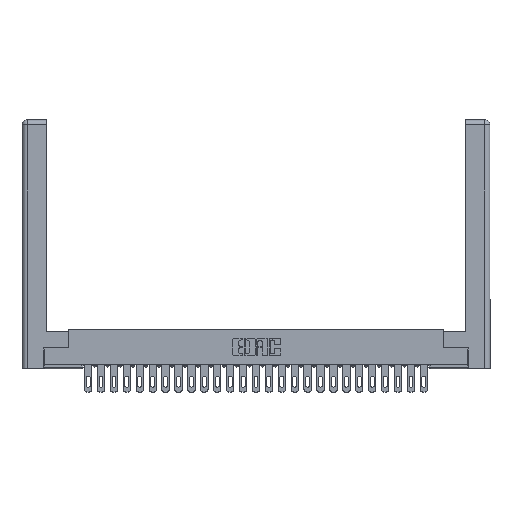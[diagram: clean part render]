
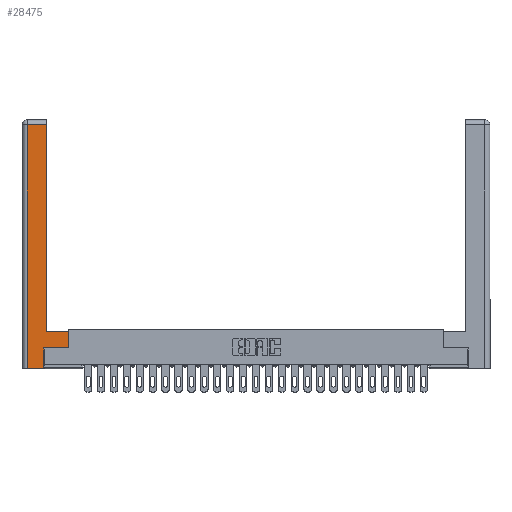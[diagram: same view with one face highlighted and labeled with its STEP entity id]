
A CAD part, top view. The second image highlights one B-rep face of the part: STEP entity #28475.
In plain terms, the highlighted planar face has unit normal (0, 0, 1).
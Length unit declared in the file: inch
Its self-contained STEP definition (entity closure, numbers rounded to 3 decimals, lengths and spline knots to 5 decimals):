
#11 = DIRECTION ( 'NONE',  ( 0., 1., 0. ) ) ;
#244 = CARTESIAN_POINT ( 'NONE',  ( 0.565, 0.245, 0. ) ) ;
#382 = ORIENTED_EDGE ( 'NONE', *, *, #28172, .T. ) ;
#699 = EDGE_CURVE ( 'NONE', #25118, #24480, #10705, .T. ) ;
#803 = CARTESIAN_POINT ( 'NONE',  ( 0.265, 0., 0. ) ) ;
#1502 = LINE ( 'NONE', #10168, #19481 ) ;
#2156 = VERTEX_POINT ( 'NONE', #7500 ) ;
#2638 = DIRECTION ( 'NONE',  ( 0., 0., -1. ) ) ;
#2921 = DIRECTION ( 'NONE',  ( -1., 0., 0. ) ) ;
#2941 = VECTOR ( 'NONE', #20913, 39.37008 ) ;
#3343 = VECTOR ( 'NONE', #12584, 39.37008 ) ;
#3544 = VECTOR ( 'NONE', #11, 39.37008 ) ;
#4178 = VECTOR ( 'NONE', #9614, 39.37008 ) ;
#4421 = LINE ( 'NONE', #15531, #13533 ) ;
#4644 = ORIENTED_EDGE ( 'NONE', *, *, #18650, .T. ) ;
#5301 = EDGE_CURVE ( 'NONE', #11600, #13776, #1502, .T. ) ;
#6294 = CARTESIAN_POINT ( 'NONE',  ( 0.565, 0.45, 0. ) ) ;
#6384 = CARTESIAN_POINT ( 'NONE',  ( 0.565, 0.45, 0. ) ) ;
#7223 = CARTESIAN_POINT ( 'NONE',  ( 0.295, 2.94, 0. ) ) ;
#7500 = CARTESIAN_POINT ( 'NONE',  ( 0.295, 0.45, 0. ) ) ;
#7998 = EDGE_CURVE ( 'NONE', #13469, #25118, #9651, .T. ) ;
#9614 = DIRECTION ( 'NONE',  ( 1., 0., 0. ) ) ;
#9651 = LINE ( 'NONE', #14152, #2941 ) ;
#10168 = CARTESIAN_POINT ( 'NONE',  ( 0.0615, 0., 0. ) ) ;
#10188 = AXIS2_PLACEMENT_3D ( 'NONE', #18360, #2638, #2921 ) ;
#10304 = CARTESIAN_POINT ( 'NONE',  ( 0.0615, 2.94, 0. ) ) ;
#10531 = VERTEX_POINT ( 'NONE', #7223 ) ;
#10705 = LINE ( 'NONE', #15296, #27817 ) ;
#11600 = VERTEX_POINT ( 'NONE', #10304 ) ;
#11806 = LINE ( 'NONE', #803, #4178 ) ;
#11919 = EDGE_CURVE ( 'NONE', #2156, #10531, #16897, .T. ) ;
#12286 = ORIENTED_EDGE ( 'NONE', *, *, #5301, .T. ) ;
#12584 = DIRECTION ( 'NONE',  ( 0., 1., 0. ) ) ;
#13469 = VERTEX_POINT ( 'NONE', #24839 ) ;
#13533 = VECTOR ( 'NONE', #19833, 39.37008 ) ;
#13776 = VERTEX_POINT ( 'NONE', #27354 ) ;
#14061 = VERTEX_POINT ( 'NONE', #6294 ) ;
#14091 = EDGE_CURVE ( 'NONE', #10531, #11600, #4421, .T. ) ;
#14152 = CARTESIAN_POINT ( 'NONE',  ( 0.265, 0.245, 0. ) ) ;
#14636 = ORIENTED_EDGE ( 'NONE', *, *, #14091, .T. ) ;
#14652 = DIRECTION ( 'NONE',  ( 0., -1., 0. ) ) ;
#15237 = EDGE_LOOP ( 'NONE', ( #25276, #14636, #12286, #382, #27289, #16051, #26134, #4644 ) ) ;
#15296 = CARTESIAN_POINT ( 'NONE',  ( 0.565, 0.245, 0. ) ) ;
#15531 = CARTESIAN_POINT ( 'NONE',  ( 0.0615, 2.94, 0. ) ) ;
#16051 = ORIENTED_EDGE ( 'NONE', *, *, #699, .T. ) ;
#16897 = LINE ( 'NONE', #25797, #3343 ) ;
#18360 = CARTESIAN_POINT ( 'NONE',  ( 0., 0., 0. ) ) ;
#18499 = PLANE ( 'NONE',  #10188 ) ;
#18650 = EDGE_CURVE ( 'NONE', #14061, #2156, #25901, .T. ) ;
#19476 = DIRECTION ( 'NONE',  ( 1., 0., 0. ) ) ;
#19481 = VECTOR ( 'NONE', #14652, 39.37008 ) ;
#19833 = DIRECTION ( 'NONE',  ( -1., 0., 0. ) ) ;
#20109 = FACE_OUTER_BOUND ( 'NONE', #15237, .T. ) ;
#20913 = DIRECTION ( 'NONE',  ( 0., 1., 0. ) ) ;
#21135 = CARTESIAN_POINT ( 'NONE',  ( 0.265, 0.245, 0. ) ) ;
#21331 = DIRECTION ( 'NONE',  ( -1., 0., 0. ) ) ;
#23773 = CARTESIAN_POINT ( 'NONE',  ( 0.295, 0.45, 0. ) ) ;
#24404 = LINE ( 'NONE', #6384, #3544 ) ;
#24480 = VERTEX_POINT ( 'NONE', #244 ) ;
#24839 = CARTESIAN_POINT ( 'NONE',  ( 0.265, 0., 0. ) ) ;
#25118 = VERTEX_POINT ( 'NONE', #21135 ) ;
#25229 = EDGE_CURVE ( 'NONE', #24480, #14061, #24404, .T. ) ;
#25276 = ORIENTED_EDGE ( 'NONE', *, *, #11919, .T. ) ;
#25570 = VECTOR ( 'NONE', #21331, 39.37008 ) ;
#25797 = CARTESIAN_POINT ( 'NONE',  ( 0.295, 3., 0. ) ) ;
#25901 = LINE ( 'NONE', #23773, #25570 ) ;
#26134 = ORIENTED_EDGE ( 'NONE', *, *, #25229, .T. ) ;
#27289 = ORIENTED_EDGE ( 'NONE', *, *, #7998, .T. ) ;
#27354 = CARTESIAN_POINT ( 'NONE',  ( 0.0615, 0., 0. ) ) ;
#27817 = VECTOR ( 'NONE', #19476, 39.37008 ) ;
#28172 = EDGE_CURVE ( 'NONE', #13776, #13469, #11806, .T. ) ;
#28475 = ADVANCED_FACE ( 'NONE', ( #20109 ), #18499, .F. ) ;
